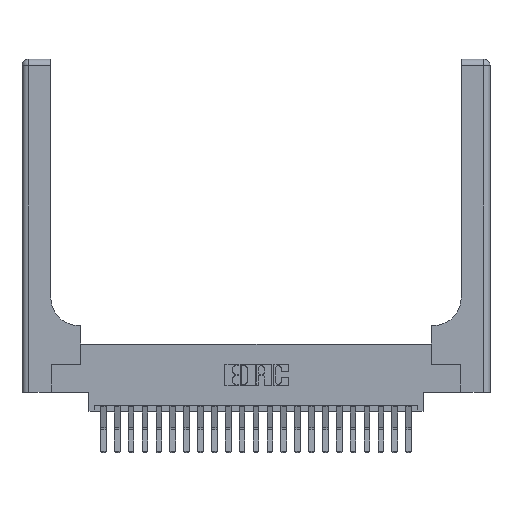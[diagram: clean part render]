
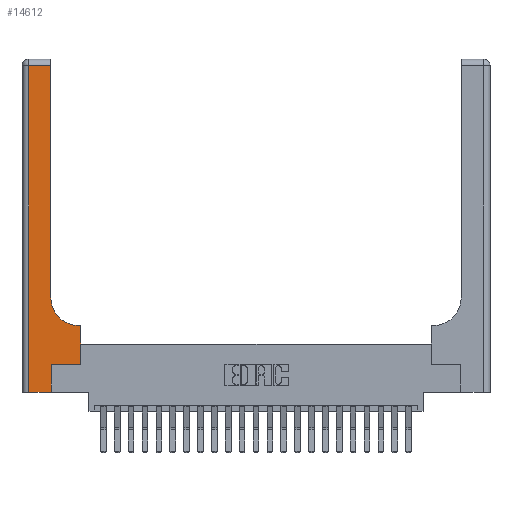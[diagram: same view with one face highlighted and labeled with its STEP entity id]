
A CAD part, top view. The second image highlights one B-rep face of the part: STEP entity #14612.
In plain terms, the highlighted planar face has unit normal (0, 0, 1).
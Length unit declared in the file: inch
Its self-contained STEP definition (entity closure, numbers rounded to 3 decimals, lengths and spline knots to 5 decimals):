
#332 = CARTESIAN_POINT ( 'NONE',  ( 0.265, 0., 0.37 ) ) ;
#489 = CARTESIAN_POINT ( 'NONE',  ( 0.265, 0., 0.37 ) ) ;
#668 = LINE ( 'NONE', #20586, #8217 ) ;
#717 = VERTEX_POINT ( 'NONE', #5434 ) ;
#780 = EDGE_CURVE ( 'NONE', #15154, #17027, #19559, .T. ) ;
#838 = DIRECTION ( 'NONE',  ( 0., 0., -1. ) ) ;
#862 = CIRCLE ( 'NONE', #20184, 0.25 ) ;
#1176 = EDGE_LOOP ( 'NONE', ( #1234, #20909, #19380, #5694, #19256, #8470, #15940, #11446, #7301 ) ) ;
#1207 = DIRECTION ( 'NONE',  ( -1., 0., 0. ) ) ;
#1234 = ORIENTED_EDGE ( 'NONE', *, *, #4480, .T. ) ;
#2030 = LINE ( 'NONE', #22801, #9141 ) ;
#2258 = AXIS2_PLACEMENT_3D ( 'NONE', #3598, #19862, #14507 ) ;
#2435 = VECTOR ( 'NONE', #1207, 39.37008 ) ;
#2834 = EDGE_CURVE ( 'NONE', #5270, #20395, #16122, .T. ) ;
#3039 = LINE ( 'NONE', #22864, #21552 ) ;
#3505 = LINE ( 'NONE', #332, #15555 ) ;
#3598 = CARTESIAN_POINT ( 'NONE',  ( 0., 3., 0.37 ) ) ;
#3682 = LINE ( 'NONE', #20058, #9003 ) ;
#4436 = EDGE_CURVE ( 'NONE', #20395, #11497, #862, .T. ) ;
#4480 = EDGE_CURVE ( 'NONE', #11497, #17079, #15974, .T. ) ;
#4593 = CARTESIAN_POINT ( 'NONE',  ( 0.06, 2.94, 0.37 ) ) ;
#4638 = VECTOR ( 'NONE', #15636, 39.37008 ) ;
#4957 = CARTESIAN_POINT ( 'NONE',  ( 0.26, 3., 0.37 ) ) ;
#5092 = EDGE_CURVE ( 'NONE', #17027, #7135, #668, .T. ) ;
#5270 = VERTEX_POINT ( 'NONE', #22841 ) ;
#5434 = CARTESIAN_POINT ( 'NONE',  ( 0.528, 0.25, 0.37 ) ) ;
#5694 = ORIENTED_EDGE ( 'NONE', *, *, #5092, .T. ) ;
#6310 = EDGE_CURVE ( 'NONE', #717, #5270, #3039, .T. ) ;
#6600 = DIRECTION ( 'NONE',  ( 0., 1., 0. ) ) ;
#7135 = VERTEX_POINT ( 'NONE', #489 ) ;
#7301 = ORIENTED_EDGE ( 'NONE', *, *, #4436, .T. ) ;
#7525 = DIRECTION ( 'NONE',  ( 0., 1., 0. ) ) ;
#8217 = VECTOR ( 'NONE', #19042, 39.37008 ) ;
#8470 = ORIENTED_EDGE ( 'NONE', *, *, #18314, .T. ) ;
#9003 = VECTOR ( 'NONE', #10918, 39.37008 ) ;
#9141 = VECTOR ( 'NONE', #15424, 39.37008 ) ;
#9161 = PLANE ( 'NONE',  #2258 ) ;
#9844 = CARTESIAN_POINT ( 'NONE',  ( 0.51, 0.85, 0.37 ) ) ;
#10918 = DIRECTION ( 'NONE',  ( -1., 0., 0. ) ) ;
#10944 = FACE_OUTER_BOUND ( 'NONE', #1176, .T. ) ;
#11362 = CARTESIAN_POINT ( 'NONE',  ( 0.265, 0.25, 0.37 ) ) ;
#11446 = ORIENTED_EDGE ( 'NONE', *, *, #2834, .T. ) ;
#11497 = VERTEX_POINT ( 'NONE', #23010 ) ;
#12203 = DIRECTION ( 'NONE',  ( 0., -1., 0. ) ) ;
#13105 = VERTEX_POINT ( 'NONE', #11362 ) ;
#14343 = EDGE_CURVE ( 'NONE', #7135, #13105, #3505, .T. ) ;
#14507 = DIRECTION ( 'NONE',  ( -1., 0., 0. ) ) ;
#14612 = ADVANCED_FACE ( 'NONE', ( #10944 ), #9161, .F. ) ;
#15140 = CARTESIAN_POINT ( 'NONE',  ( 0.51, 0.6, 0.37 ) ) ;
#15154 = VERTEX_POINT ( 'NONE', #4593 ) ;
#15424 = DIRECTION ( 'NONE',  ( 1., 0., 0. ) ) ;
#15555 = VECTOR ( 'NONE', #7525, 39.37008 ) ;
#15636 = DIRECTION ( 'NONE',  ( 0., 1., 0. ) ) ;
#15940 = ORIENTED_EDGE ( 'NONE', *, *, #6310, .T. ) ;
#15974 = LINE ( 'NONE', #4957, #4638 ) ;
#16122 = LINE ( 'NONE', #23148, #2435 ) ;
#16224 = EDGE_CURVE ( 'NONE', #17079, #15154, #3682, .T. ) ;
#17027 = VERTEX_POINT ( 'NONE', #18202 ) ;
#17079 = VERTEX_POINT ( 'NONE', #17757 ) ;
#17757 = CARTESIAN_POINT ( 'NONE',  ( 0.26, 2.94, 0.37 ) ) ;
#18202 = CARTESIAN_POINT ( 'NONE',  ( 0.06, 0., 0.37 ) ) ;
#18314 = EDGE_CURVE ( 'NONE', #13105, #717, #2030, .T. ) ;
#19042 = DIRECTION ( 'NONE',  ( 1., 0., 0. ) ) ;
#19256 = ORIENTED_EDGE ( 'NONE', *, *, #14343, .T. ) ;
#19380 = ORIENTED_EDGE ( 'NONE', *, *, #780, .T. ) ;
#19427 = VECTOR ( 'NONE', #12203, 39.37008 ) ;
#19441 = CARTESIAN_POINT ( 'NONE',  ( 0.06, 3., 0.37 ) ) ;
#19559 = LINE ( 'NONE', #19441, #19427 ) ;
#19862 = DIRECTION ( 'NONE',  ( 0., 0., -1. ) ) ;
#20058 = CARTESIAN_POINT ( 'NONE',  ( 0., 2.94, 0.37 ) ) ;
#20184 = AXIS2_PLACEMENT_3D ( 'NONE', #9844, #838, #22549 ) ;
#20395 = VERTEX_POINT ( 'NONE', #15140 ) ;
#20586 = CARTESIAN_POINT ( 'NONE',  ( 0., 0., 0.37 ) ) ;
#20909 = ORIENTED_EDGE ( 'NONE', *, *, #16224, .T. ) ;
#21552 = VECTOR ( 'NONE', #6600, 39.37008 ) ;
#22549 = DIRECTION ( 'NONE',  ( 1., 0., 0. ) ) ;
#22801 = CARTESIAN_POINT ( 'NONE',  ( 0.265, 0.25, 0.37 ) ) ;
#22841 = CARTESIAN_POINT ( 'NONE',  ( 0.528, 0.6, 0.37 ) ) ;
#22864 = CARTESIAN_POINT ( 'NONE',  ( 0.528, 0.25, 0.37 ) ) ;
#23010 = CARTESIAN_POINT ( 'NONE',  ( 0.26, 0.85, 0.37 ) ) ;
#23148 = CARTESIAN_POINT ( 'NONE',  ( 0.26, 0.6, 0.37 ) ) ;
